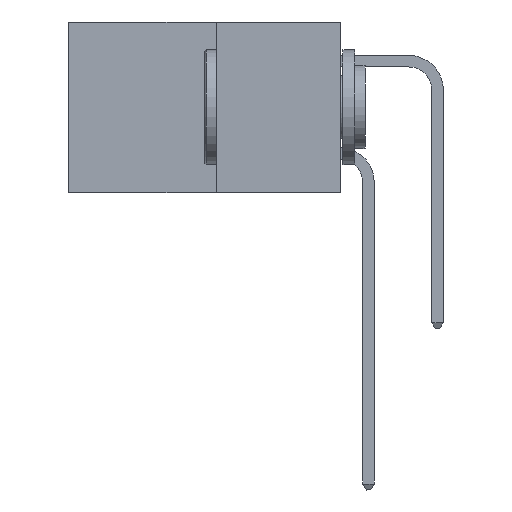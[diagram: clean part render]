
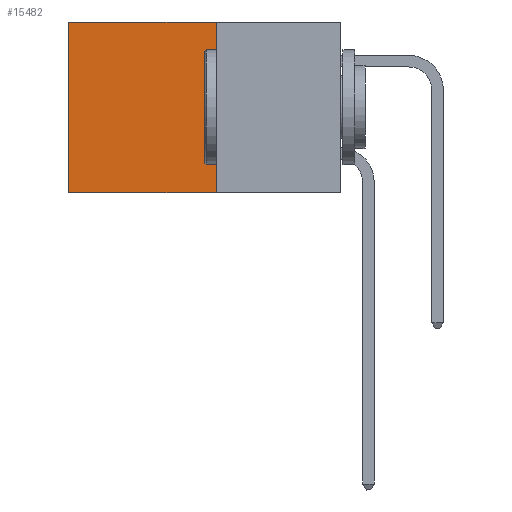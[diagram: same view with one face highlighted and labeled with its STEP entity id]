
A CAD part, left-side view. The second image highlights one B-rep face of the part: STEP entity #15482.
In plain terms, the highlighted planar face has unit normal (-1, 0, 0).
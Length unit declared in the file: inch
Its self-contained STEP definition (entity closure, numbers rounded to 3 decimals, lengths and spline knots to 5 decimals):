
#430 = AXIS2_PLACEMENT_3D ( 'NONE', #4755, #19696, #8592 ) ;
#905 = LINE ( 'NONE', #3678, #10433 ) ;
#984 = VECTOR ( 'NONE', #6664, 39.37008 ) ;
#1151 = LINE ( 'NONE', #18366, #5651 ) ;
#2299 = VERTEX_POINT ( 'NONE', #7550 ) ;
#2353 = EDGE_LOOP ( 'NONE', ( #20475, #9469, #4730, #11911 ) ) ;
#2533 = CARTESIAN_POINT ( 'NONE',  ( 0.277, 0.59, -0.37 ) ) ;
#3412 = VERTEX_POINT ( 'NONE', #2533 ) ;
#3678 = CARTESIAN_POINT ( 'NONE',  ( 0.277, 0.27, -0.37 ) ) ;
#3766 = VERTEX_POINT ( 'NONE', #22767 ) ;
#4730 = ORIENTED_EDGE ( 'NONE', *, *, #17891, .F. ) ;
#4755 = CARTESIAN_POINT ( 'NONE',  ( 0.277, 0.27, -0.37 ) ) ;
#5651 = VECTOR ( 'NONE', #20263, 39.37008 ) ;
#6098 = LINE ( 'NONE', #15941, #984 ) ;
#6664 = DIRECTION ( 'NONE',  ( 0., 1., 0. ) ) ;
#6692 = PLANE ( 'NONE',  #430 ) ;
#7299 = DIRECTION ( 'NONE',  ( 0., 0., -1. ) ) ;
#7550 = CARTESIAN_POINT ( 'NONE',  ( 0.277, 0.27, 0. ) ) ;
#7688 = VECTOR ( 'NONE', #7299, 39.37008 ) ;
#8592 = DIRECTION ( 'NONE',  ( 0., 0., -1. ) ) ;
#9469 = ORIENTED_EDGE ( 'NONE', *, *, #19355, .F. ) ;
#10103 = CARTESIAN_POINT ( 'NONE',  ( 0.277, 0.27, -0.37 ) ) ;
#10350 = EDGE_CURVE ( 'NONE', #3766, #3412, #18125, .T. ) ;
#10433 = VECTOR ( 'NONE', #11207, 39.37008 ) ;
#11207 = DIRECTION ( 'NONE',  ( 0., 0., -1. ) ) ;
#11911 = ORIENTED_EDGE ( 'NONE', *, *, #13744, .T. ) ;
#13744 = EDGE_CURVE ( 'NONE', #2299, #3766, #1151, .T. ) ;
#15482 = ADVANCED_FACE ( 'NONE', ( #16063 ), #6692, .F. ) ;
#15941 = CARTESIAN_POINT ( 'NONE',  ( 0.277, 0.27, -0.37 ) ) ;
#16063 = FACE_OUTER_BOUND ( 'NONE', #2353, .T. ) ;
#17891 = EDGE_CURVE ( 'NONE', #2299, #23030, #905, .T. ) ;
#18125 = LINE ( 'NONE', #23908, #7688 ) ;
#18366 = CARTESIAN_POINT ( 'NONE',  ( 0.277, 0.27, 0. ) ) ;
#19355 = EDGE_CURVE ( 'NONE', #23030, #3412, #6098, .T. ) ;
#19696 = DIRECTION ( 'NONE',  ( 1., 0., 0. ) ) ;
#20263 = DIRECTION ( 'NONE',  ( 0., 1., 0. ) ) ;
#20475 = ORIENTED_EDGE ( 'NONE', *, *, #10350, .T. ) ;
#22767 = CARTESIAN_POINT ( 'NONE',  ( 0.277, 0.59, 0. ) ) ;
#23030 = VERTEX_POINT ( 'NONE', #10103 ) ;
#23908 = CARTESIAN_POINT ( 'NONE',  ( 0.277, 0.59, -0.37 ) ) ;
